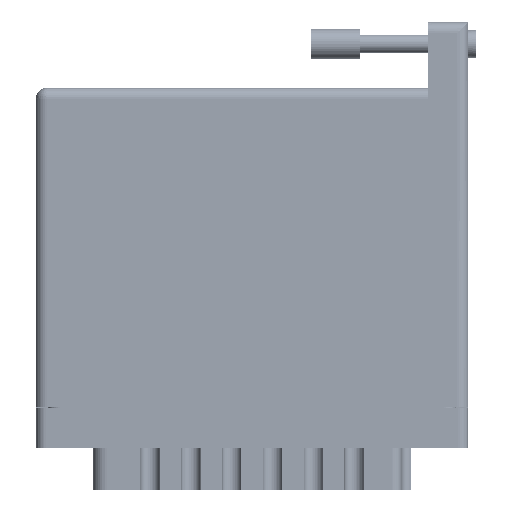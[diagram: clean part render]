
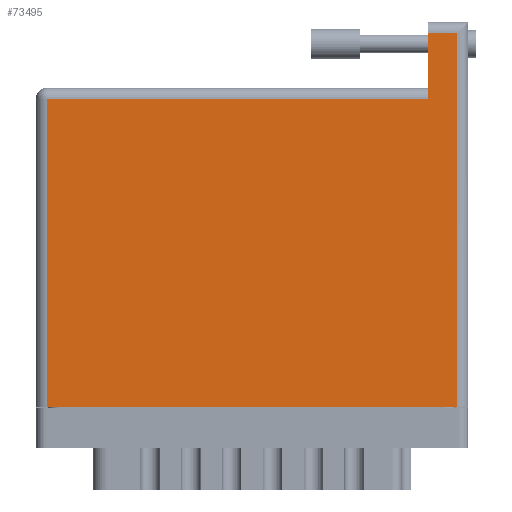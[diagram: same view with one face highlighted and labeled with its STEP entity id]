
A CAD part, front view. The second image highlights one B-rep face of the part: STEP entity #73495.
In plain terms, the highlighted face is planar.
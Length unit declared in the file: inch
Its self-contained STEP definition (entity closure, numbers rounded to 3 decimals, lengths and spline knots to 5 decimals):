
#19 = VERTEX_POINT ( 'NONE', #43022 ) ;
#212 = ORIENTED_EDGE ( 'NONE', *, *, #84748, .T. ) ;
#246 = EDGE_CURVE ( 'NONE', #62258, #3011, #13455, .T. ) ;
#3011 = VERTEX_POINT ( 'NONE', #79837 ) ;
#5175 = VECTOR ( 'NONE', #12384, 39.37008 ) ;
#6640 = DIRECTION ( 'NONE',  ( 1., 0., 0. ) ) ;
#7423 = ORIENTED_EDGE ( 'NONE', *, *, #61059, .T. ) ;
#9488 = CARTESIAN_POINT ( 'NONE',  ( 0.07, 0., 0. ) ) ;
#11656 = CARTESIAN_POINT ( 'NONE',  ( 2.685, 2.45, 0. ) ) ;
#12384 = DIRECTION ( 'NONE',  ( 0., -1., 0. ) ) ;
#13257 = ORIENTED_EDGE ( 'NONE', *, *, #246, .T. ) ;
#13324 = CARTESIAN_POINT ( 'NONE',  ( 2.499, 2.45, 0. ) ) ;
#13455 = LINE ( 'NONE', #51807, #29760 ) ;
#14174 = CARTESIAN_POINT ( 'NONE',  ( 2.499, 1.96, 0. ) ) ;
#14885 = AXIS2_PLACEMENT_3D ( 'NONE', #59133, #37274, #52273 ) ;
#17032 = VERTEX_POINT ( 'NONE', #14174 ) ;
#20230 = CARTESIAN_POINT ( 'NONE',  ( 0.07, 0., 0. ) ) ;
#25242 = VECTOR ( 'NONE', #44310, 39.37008 ) ;
#29760 = VECTOR ( 'NONE', #6640, 39.37008 ) ;
#30710 = LINE ( 'NONE', #11656, #43476 ) ;
#30753 = LINE ( 'NONE', #20230, #79753 ) ;
#37274 = DIRECTION ( 'NONE',  ( 0., 0., -1. ) ) ;
#37783 = CARTESIAN_POINT ( 'NONE',  ( 0., 1.96, 0. ) ) ;
#41308 = ORIENTED_EDGE ( 'NONE', *, *, #75361, .T. ) ;
#43022 = CARTESIAN_POINT ( 'NONE',  ( 2.499, 2.38, 0. ) ) ;
#43476 = VECTOR ( 'NONE', #48013, 39.37008 ) ;
#44310 = DIRECTION ( 'NONE',  ( -1., 0., 0. ) ) ;
#45720 = VERTEX_POINT ( 'NONE', #51588 ) ;
#46279 = ORIENTED_EDGE ( 'NONE', *, *, #81958, .T. ) ;
#48013 = DIRECTION ( 'NONE',  ( 0., 1., 0. ) ) ;
#48039 = VECTOR ( 'NONE', #55953, 39.37008 ) ;
#51588 = CARTESIAN_POINT ( 'NONE',  ( 2.685, 2.38, 0. ) ) ;
#51807 = CARTESIAN_POINT ( 'NONE',  ( 0., 0., 0. ) ) ;
#52273 = DIRECTION ( 'NONE',  ( -1., 0., 0. ) ) ;
#55953 = DIRECTION ( 'NONE',  ( -1., 0., 0. ) ) ;
#59133 = CARTESIAN_POINT ( 'NONE',  ( 0., 2.03, 0. ) ) ;
#61059 = EDGE_CURVE ( 'NONE', #45720, #19, #73713, .T. ) ;
#61343 = ORIENTED_EDGE ( 'NONE', *, *, #63241, .T. ) ;
#61365 = FACE_OUTER_BOUND ( 'NONE', #80028, .T. ) ;
#62258 = VERTEX_POINT ( 'NONE', #9488 ) ;
#63241 = EDGE_CURVE ( 'NONE', #65210, #62258, #30753, .T. ) ;
#65210 = VERTEX_POINT ( 'NONE', #68520 ) ;
#68520 = CARTESIAN_POINT ( 'NONE',  ( 0.07, 1.96, 0. ) ) ;
#73017 = LINE ( 'NONE', #37783, #25242 ) ;
#73495 = ADVANCED_FACE ( 'NONE', ( #61365 ), #89414, .F. ) ;
#73713 = LINE ( 'NONE', #93086, #48039 ) ;
#75361 = EDGE_CURVE ( 'NONE', #3011, #45720, #30710, .T. ) ;
#78557 = LINE ( 'NONE', #13324, #5175 ) ;
#79753 = VECTOR ( 'NONE', #95415, 39.37008 ) ;
#79837 = CARTESIAN_POINT ( 'NONE',  ( 2.685, 0., 0. ) ) ;
#80028 = EDGE_LOOP ( 'NONE', ( #46279, #212, #61343, #13257, #41308, #7423 ) ) ;
#81958 = EDGE_CURVE ( 'NONE', #19, #17032, #78557, .T. ) ;
#84748 = EDGE_CURVE ( 'NONE', #17032, #65210, #73017, .T. ) ;
#89414 = PLANE ( 'NONE',  #14885 ) ;
#93086 = CARTESIAN_POINT ( 'NONE',  ( 0., 2.38, 0. ) ) ;
#95415 = DIRECTION ( 'NONE',  ( 0., -1., 0. ) ) ;
